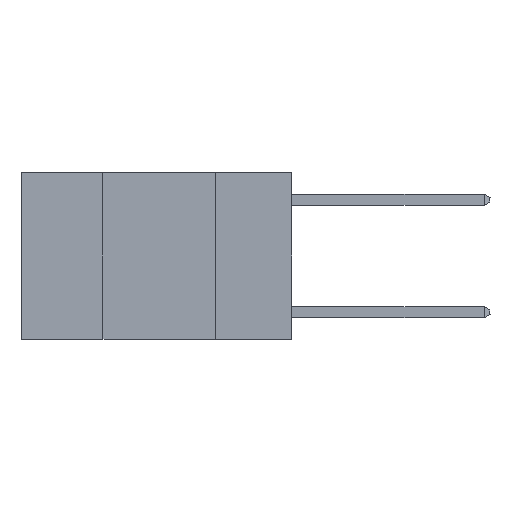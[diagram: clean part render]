
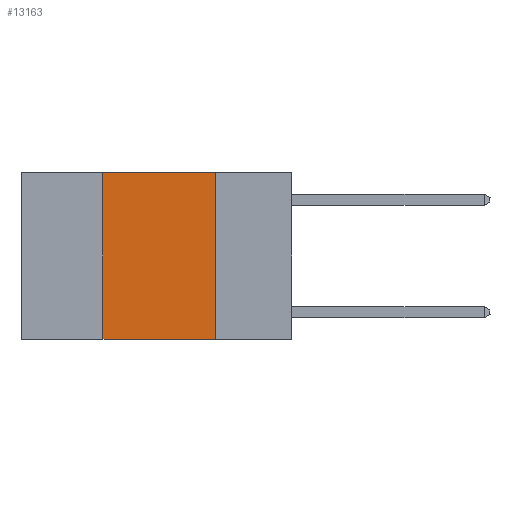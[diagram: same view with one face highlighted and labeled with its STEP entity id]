
A CAD part, left-side view. The second image highlights one B-rep face of the part: STEP entity #13163.
In plain terms, the highlighted planar face has unit normal (-1, 0, 0).
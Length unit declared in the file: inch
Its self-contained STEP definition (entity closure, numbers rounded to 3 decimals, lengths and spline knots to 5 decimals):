
#59 = DIRECTION ( 'NONE',  ( 0., -1., 0. ) ) ;
#457 = EDGE_CURVE ( 'NONE', #4166, #2899, #1263, .T. ) ;
#736 = VERTEX_POINT ( 'NONE', #5681 ) ;
#870 = VERTEX_POINT ( 'NONE', #13273 ) ;
#1263 = LINE ( 'NONE', #2618, #3101 ) ;
#1462 = EDGE_LOOP ( 'NONE', ( #8914, #12954, #4002, #7517 ) ) ;
#2222 = DIRECTION ( 'NONE',  ( 1., 0., 0. ) ) ;
#2618 = CARTESIAN_POINT ( 'NONE',  ( 0., 0.6, 0. ) ) ;
#2690 = LINE ( 'NONE', #9828, #15066 ) ;
#2892 = VECTOR ( 'NONE', #10610, 39.37008 ) ;
#2899 = VERTEX_POINT ( 'NONE', #8529 ) ;
#2988 = EDGE_CURVE ( 'NONE', #2899, #870, #8610, .T. ) ;
#3101 = VECTOR ( 'NONE', #59, 39.37008 ) ;
#3479 = VECTOR ( 'NONE', #4263, 39.37008 ) ;
#4002 = ORIENTED_EDGE ( 'NONE', *, *, #12069, .F. ) ;
#4166 = VERTEX_POINT ( 'NONE', #4532 ) ;
#4263 = DIRECTION ( 'NONE',  ( 0., 0., -1. ) ) ;
#4532 = CARTESIAN_POINT ( 'NONE',  ( 0., 0.42, 0. ) ) ;
#5681 = CARTESIAN_POINT ( 'NONE',  ( 0., 0.42, -0.37 ) ) ;
#6920 = CARTESIAN_POINT ( 'NONE',  ( 0., 0.6, -0.37 ) ) ;
#7517 = ORIENTED_EDGE ( 'NONE', *, *, #14285, .T. ) ;
#8374 = PLANE ( 'NONE',  #13143 ) ;
#8529 = CARTESIAN_POINT ( 'NONE',  ( 0., 0.17, 0. ) ) ;
#8610 = LINE ( 'NONE', #13281, #3479 ) ;
#8914 = ORIENTED_EDGE ( 'NONE', *, *, #2988, .F. ) ;
#9465 = CARTESIAN_POINT ( 'NONE',  ( 0., 0.6, 0. ) ) ;
#9828 = CARTESIAN_POINT ( 'NONE',  ( 0., 0.42, 0. ) ) ;
#10610 = DIRECTION ( 'NONE',  ( 0., -1., 0. ) ) ;
#12069 = EDGE_CURVE ( 'NONE', #736, #4166, #2690, .T. ) ;
#12954 = ORIENTED_EDGE ( 'NONE', *, *, #457, .F. ) ;
#13143 = AXIS2_PLACEMENT_3D ( 'NONE', #9465, #2222, #15336 ) ;
#13163 = ADVANCED_FACE ( 'NONE', ( #15259 ), #8374, .F. ) ;
#13273 = CARTESIAN_POINT ( 'NONE',  ( 0., 0.17, -0.37 ) ) ;
#13281 = CARTESIAN_POINT ( 'NONE',  ( 0., 0.17, 0. ) ) ;
#14222 = LINE ( 'NONE', #6920, #2892 ) ;
#14285 = EDGE_CURVE ( 'NONE', #736, #870, #14222, .T. ) ;
#14639 = DIRECTION ( 'NONE',  ( 0., 0., 1. ) ) ;
#15066 = VECTOR ( 'NONE', #14639, 39.37008 ) ;
#15259 = FACE_OUTER_BOUND ( 'NONE', #1462, .T. ) ;
#15336 = DIRECTION ( 'NONE',  ( 0., 0., -1. ) ) ;
